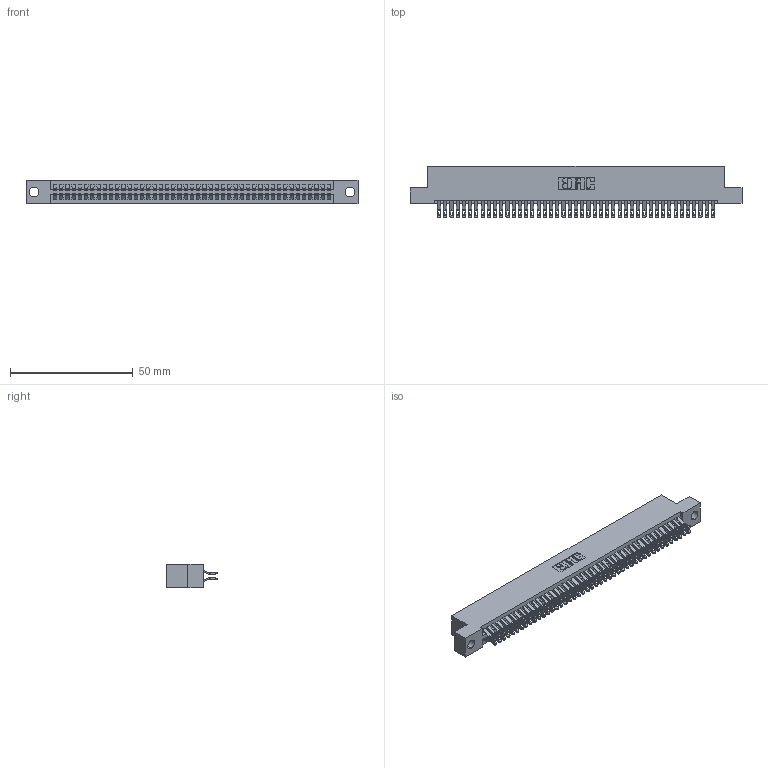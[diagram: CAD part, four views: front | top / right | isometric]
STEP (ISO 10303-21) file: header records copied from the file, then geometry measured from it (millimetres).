
FILE_DESCRIPTION (( 'STEP AP203' ), '1' );
FILE_NAME ('395-090-555-204.STEP', '2021-06-17T10:16:53', ( '' ), ( '' ), 'SwSTEP 2.0', 'SolidWorks 2020', '' );
FILE_SCHEMA (( 'CONFIG_CONTROL_DESIGN' ));
Length unit declared in the file: inch
Products named in the file (3): 395-090-555-204; 345-292-001_555 Tail; 345 Part_Flush Mounting Lugs - 0.156 Dia-TI
Assembly tree (91 placements, depth 2):
  395-090-555-204
    345 Part_Flush Mounting Lugs - 0.156 Dia-TI
    345-292-001_555 Tail  x90
Bounding box: 135.51 x 21.13 x 9.4 mm (x, y, z)
Volume: 13346.4 mm3; surface area: 20545.9 mm2
Topology: 91 solids, 91 shells, 5180 faces, 16307 edges, 10870 vertices
Faces by surface type: plane 2884, cylinder 2296
Entity records: 35649 total; most frequent: CARTESIAN_POINT 6012, ORIENTED_EDGE 5914, DIRECTION 5265, EDGE_CURVE 2957, LINE 2625, VECTOR 2625, VERTEX_POINT 1970, AXIS2_PLACEMENT_3D 1320
